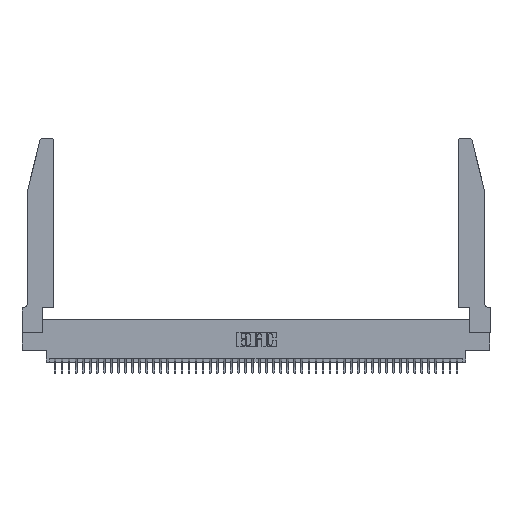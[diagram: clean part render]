
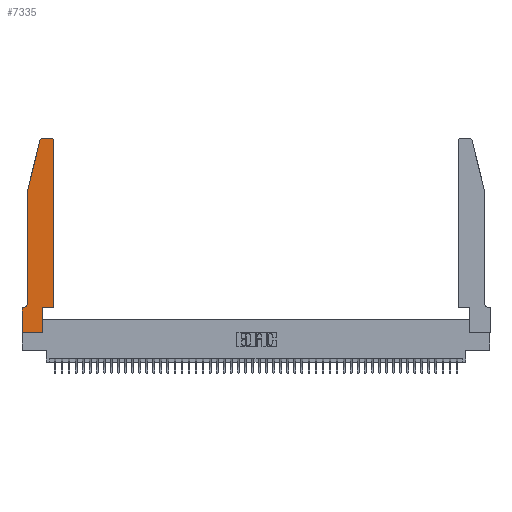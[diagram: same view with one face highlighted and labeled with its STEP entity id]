
A CAD part, top view. The second image highlights one B-rep face of the part: STEP entity #7335.
In plain terms, the highlighted planar face has unit normal (0, 0, 1).
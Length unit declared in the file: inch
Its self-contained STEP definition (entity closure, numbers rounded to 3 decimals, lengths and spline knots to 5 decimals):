
#1606 = EDGE_CURVE ( 'NONE', #4731, #2614, #2343, .T. ) ;
#1879 = EDGE_CURVE ( 'NONE', #2614, #3403, #22926, .T. ) ;
#2343 = LINE ( 'NONE', #40221, #22364 ) ;
#2420 = ORIENTED_EDGE ( 'NONE', *, *, #36559, .T. ) ;
#2614 = VERTEX_POINT ( 'NONE', #11691 ) ;
#2820 = DIRECTION ( 'NONE',  ( 1., 0., 0. ) ) ;
#2837 = ORIENTED_EDGE ( 'NONE', *, *, #31916, .T. ) ;
#3139 = CARTESIAN_POINT ( 'NONE',  ( 0., 0.35, 0.37 ) ) ;
#3403 = VERTEX_POINT ( 'NONE', #25954 ) ;
#3693 = CIRCLE ( 'NONE', #41257, 0.03 ) ;
#3995 = DIRECTION ( 'NONE',  ( 0., -1., 0. ) ) ;
#4731 = VERTEX_POINT ( 'NONE', #34357 ) ;
#5085 = ORIENTED_EDGE ( 'NONE', *, *, #1879, .T. ) ;
#6645 = CARTESIAN_POINT ( 'NONE',  ( 0.0755, 2., 0.37 ) ) ;
#6672 = DIRECTION ( 'NONE',  ( 0., 1., 0. ) ) ;
#6697 = DIRECTION ( 'NONE',  ( -1., 0., 0. ) ) ;
#7335 = ADVANCED_FACE ( 'NONE', ( #39210 ), #29209, .T. ) ;
#7376 = VERTEX_POINT ( 'NONE', #19793 ) ;
#8270 = VERTEX_POINT ( 'NONE', #14053 ) ;
#8575 = VECTOR ( 'NONE', #13182, 39.37008 ) ;
#11072 = CARTESIAN_POINT ( 'NONE',  ( 0., 0., 0.37 ) ) ;
#11614 = CARTESIAN_POINT ( 'NONE',  ( 0.4505, 0.35, 0.37 ) ) ;
#11690 = EDGE_CURVE ( 'NONE', #24606, #7376, #41847, .T. ) ;
#11691 = CARTESIAN_POINT ( 'NONE',  ( 0.2865, 0.35, 0.37 ) ) ;
#11933 = ORIENTED_EDGE ( 'NONE', *, *, #17592, .T. ) ;
#12081 = CARTESIAN_POINT ( 'NONE',  ( 0.4205, 2.72, 0.37 ) ) ;
#12216 = VERTEX_POINT ( 'NONE', #13857 ) ;
#12386 = AXIS2_PLACEMENT_3D ( 'NONE', #3139, #25297, #2820 ) ;
#12662 = EDGE_CURVE ( 'NONE', #3403, #46866, #19681, .T. ) ;
#12739 = DIRECTION ( 'NONE',  ( 0., 0., 1. ) ) ;
#13182 = DIRECTION ( 'NONE',  ( -1., 0., 0. ) ) ;
#13227 = ORIENTED_EDGE ( 'NONE', *, *, #34857, .T. ) ;
#13415 = VECTOR ( 'NONE', #33703, 39.37008 ) ;
#13857 = CARTESIAN_POINT ( 'NONE',  ( 0.0755, 0.42, 0.37 ) ) ;
#14053 = CARTESIAN_POINT ( 'NONE',  ( 0., 0.35, 0.37 ) ) ;
#14113 = VECTOR ( 'NONE', #17932, 39.37008 ) ;
#15627 = CARTESIAN_POINT ( 'NONE',  ( 0.4205, 2.75, 0.37 ) ) ;
#15873 = CARTESIAN_POINT ( 'NONE',  ( 0.0755, 2., 0.37 ) ) ;
#16608 = AXIS2_PLACEMENT_3D ( 'NONE', #25245, #28664, #6697 ) ;
#16901 = LINE ( 'NONE', #15873, #24498 ) ;
#17176 = CARTESIAN_POINT ( 'NONE',  ( 0.0755, 0.35, 0.37 ) ) ;
#17592 = EDGE_CURVE ( 'NONE', #19234, #8270, #33165, .T. ) ;
#17885 = CARTESIAN_POINT ( 'NONE',  ( 0.4505, 2.72, 0.37 ) ) ;
#17932 = DIRECTION ( 'NONE',  ( 1., 0., 0. ) ) ;
#18556 = AXIS2_PLACEMENT_3D ( 'NONE', #39308, #31352, #42417 ) ;
#19097 = VECTOR ( 'NONE', #29588, 39.37008 ) ;
#19234 = VERTEX_POINT ( 'NONE', #42476 ) ;
#19681 = LINE ( 'NONE', #11614, #23777 ) ;
#19793 = CARTESIAN_POINT ( 'NONE',  ( 0.0755, 2., 0.37 ) ) ;
#19959 = DIRECTION ( 'NONE',  ( 0., -1., 0. ) ) ;
#20336 = DIRECTION ( 'NONE',  ( -1., 0., 0. ) ) ;
#20822 = ORIENTED_EDGE ( 'NONE', *, *, #11690, .T. ) ;
#21431 = ORIENTED_EDGE ( 'NONE', *, *, #1606, .T. ) ;
#22364 = VECTOR ( 'NONE', #6672, 39.37008 ) ;
#22800 = DIRECTION ( 'NONE',  ( 0., 1., 0. ) ) ;
#22926 = LINE ( 'NONE', #29195, #14113 ) ;
#23777 = VECTOR ( 'NONE', #22800, 39.37008 ) ;
#24498 = VECTOR ( 'NONE', #19959, 39.37008 ) ;
#24606 = VERTEX_POINT ( 'NONE', #46315 ) ;
#25245 = CARTESIAN_POINT ( 'NONE',  ( 0.0055, 0.42, 0.37 ) ) ;
#25297 = DIRECTION ( 'NONE',  ( 0., 0., 1. ) ) ;
#25351 = CIRCLE ( 'NONE', #16608, 0.07 ) ;
#25954 = CARTESIAN_POINT ( 'NONE',  ( 0.4505, 0.35, 0.37 ) ) ;
#26199 = LINE ( 'NONE', #39016, #8575 ) ;
#26347 = CARTESIAN_POINT ( 'NONE',  ( 0., 0., 0.37 ) ) ;
#27706 = EDGE_LOOP ( 'NONE', ( #31697, #28952, #20822, #2837, #44645, #11933, #2420, #36971, #21431, #5085, #46106, #13227 ) ) ;
#28055 = VERTEX_POINT ( 'NONE', #11072 ) ;
#28664 = DIRECTION ( 'NONE',  ( 0., 0., -1. ) ) ;
#28907 = VERTEX_POINT ( 'NONE', #15627 ) ;
#28952 = ORIENTED_EDGE ( 'NONE', *, *, #39761, .T. ) ;
#29195 = CARTESIAN_POINT ( 'NONE',  ( 0.4505, 0.35, 0.37 ) ) ;
#29209 = PLANE ( 'NONE',  #12386 ) ;
#29588 = DIRECTION ( 'NONE',  ( -0.239, -0.971, 0. ) ) ;
#29630 = VECTOR ( 'NONE', #20336, 39.37008 ) ;
#30414 = CARTESIAN_POINT ( 'NONE',  ( 0., 0., 0.37 ) ) ;
#31352 = DIRECTION ( 'NONE',  ( 0., 0., 1. ) ) ;
#31697 = ORIENTED_EDGE ( 'NONE', *, *, #45531, .T. ) ;
#31717 = EDGE_CURVE ( 'NONE', #28055, #4731, #46102, .T. ) ;
#31916 = EDGE_CURVE ( 'NONE', #7376, #12216, #16901, .T. ) ;
#32206 = CIRCLE ( 'NONE', #18556, 0.03 ) ;
#32305 = VECTOR ( 'NONE', #3995, 39.37008 ) ;
#33165 = LINE ( 'NONE', #17176, #29630 ) ;
#33703 = DIRECTION ( 'NONE',  ( 1., 0., 0. ) ) ;
#34357 = CARTESIAN_POINT ( 'NONE',  ( 0.2865, 0., 0.37 ) ) ;
#34857 = EDGE_CURVE ( 'NONE', #46866, #28907, #3693, .T. ) ;
#35154 = DIRECTION ( 'NONE',  ( 1., 0., 0. ) ) ;
#36038 = CARTESIAN_POINT ( 'NONE',  ( 0.284, 2.75, 0.37 ) ) ;
#36559 = EDGE_CURVE ( 'NONE', #8270, #28055, #36981, .T. ) ;
#36971 = ORIENTED_EDGE ( 'NONE', *, *, #31717, .T. ) ;
#36981 = LINE ( 'NONE', #30414, #32305 ) ;
#38051 = EDGE_CURVE ( 'NONE', #12216, #19234, #25351, .T. ) ;
#38112 = VERTEX_POINT ( 'NONE', #36038 ) ;
#39016 = CARTESIAN_POINT ( 'NONE',  ( 0.2605, 2.75, 0.37 ) ) ;
#39210 = FACE_OUTER_BOUND ( 'NONE', #27706, .T. ) ;
#39308 = CARTESIAN_POINT ( 'NONE',  ( 0.284, 2.72, 0.37 ) ) ;
#39761 = EDGE_CURVE ( 'NONE', #38112, #24606, #32206, .T. ) ;
#40221 = CARTESIAN_POINT ( 'NONE',  ( 0.2865, 0.35, 0.37 ) ) ;
#41257 = AXIS2_PLACEMENT_3D ( 'NONE', #12081, #12739, #35154 ) ;
#41847 = LINE ( 'NONE', #6645, #19097 ) ;
#42417 = DIRECTION ( 'NONE',  ( 1., 0., 0. ) ) ;
#42476 = CARTESIAN_POINT ( 'NONE',  ( 0.0055, 0.35, 0.37 ) ) ;
#44645 = ORIENTED_EDGE ( 'NONE', *, *, #38051, .T. ) ;
#45531 = EDGE_CURVE ( 'NONE', #28907, #38112, #26199, .T. ) ;
#46102 = LINE ( 'NONE', #26347, #13415 ) ;
#46106 = ORIENTED_EDGE ( 'NONE', *, *, #12662, .T. ) ;
#46315 = CARTESIAN_POINT ( 'NONE',  ( 0.25487, 2.72718, 0.37 ) ) ;
#46866 = VERTEX_POINT ( 'NONE', #17885 ) ;
